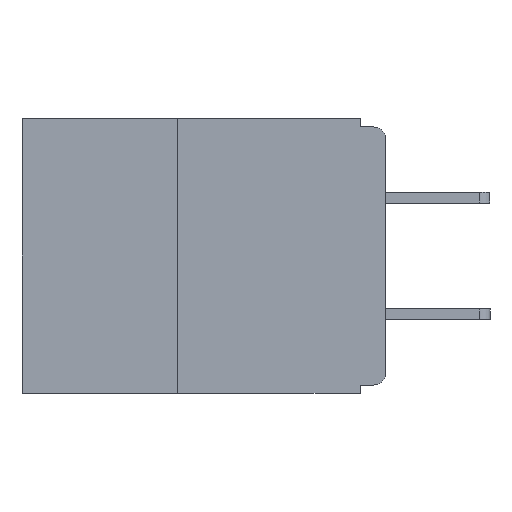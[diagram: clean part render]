
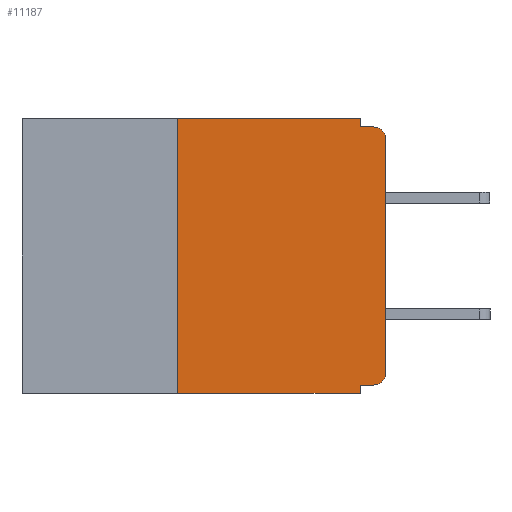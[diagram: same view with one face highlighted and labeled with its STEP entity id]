
A CAD part, left-side view. The second image highlights one B-rep face of the part: STEP entity #11187.
In plain terms, the highlighted planar face has unit normal (-1, 0, 0).
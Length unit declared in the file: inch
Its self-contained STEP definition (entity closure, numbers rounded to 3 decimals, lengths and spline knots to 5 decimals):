
#451 = EDGE_CURVE ( 'NONE', #9233, #1102, #5130, .T. ) ;
#1060 = CARTESIAN_POINT ( 'NONE',  ( 0., 0.437, 0. ) ) ;
#1102 = VERTEX_POINT ( 'NONE', #16081 ) ;
#1168 = VERTEX_POINT ( 'NONE', #16464 ) ;
#1625 = EDGE_LOOP ( 'NONE', ( #16126, #7980, #3937, #9539, #2246, #13802, #11364, #14177, #5556, #2811 ) ) ;
#1728 = EDGE_CURVE ( 'NONE', #16707, #11199, #4581, .T. ) ;
#2154 = LINE ( 'NONE', #1060, #18234 ) ;
#2246 = ORIENTED_EDGE ( 'NONE', *, *, #17163, .F. ) ;
#2491 = CARTESIAN_POINT ( 'NONE',  ( 0., 0.015, -0.32 ) ) ;
#2811 = ORIENTED_EDGE ( 'NONE', *, *, #14658, .T. ) ;
#3799 = CARTESIAN_POINT ( 'NONE',  ( 0., 0.015, -0.305 ) ) ;
#3903 = CARTESIAN_POINT ( 'NONE',  ( 0., 0., -0.01 ) ) ;
#3937 = ORIENTED_EDGE ( 'NONE', *, *, #18074, .F. ) ;
#4063 = DIRECTION ( 'NONE',  ( -1., 0., 0. ) ) ;
#4570 = DIRECTION ( 'NONE',  ( 0., 0., -1. ) ) ;
#4581 = LINE ( 'NONE', #18368, #12047 ) ;
#4763 = DIRECTION ( 'NONE',  ( 0., 0., -1. ) ) ;
#4775 = CARTESIAN_POINT ( 'NONE',  ( 0., 0.031, 0. ) ) ;
#4982 = CARTESIAN_POINT ( 'NONE',  ( 0., 0.015, -0.025 ) ) ;
#5008 = CARTESIAN_POINT ( 'NONE',  ( 0., 0., 0. ) ) ;
#5130 = LINE ( 'NONE', #5008, #12098 ) ;
#5236 = CARTESIAN_POINT ( 'NONE',  ( 0., 0., -0.305 ) ) ;
#5355 = DIRECTION ( 'NONE',  ( 0., 0., -1. ) ) ;
#5543 = LINE ( 'NONE', #8065, #14259 ) ;
#5556 = ORIENTED_EDGE ( 'NONE', *, *, #9085, .F. ) ;
#6046 = LINE ( 'NONE', #4775, #13821 ) ;
#6303 = CARTESIAN_POINT ( 'NONE',  ( 0., 0.25, -0.33 ) ) ;
#6414 = DIRECTION ( 'NONE',  ( 0., 0., 1. ) ) ;
#6687 = CARTESIAN_POINT ( 'NONE',  ( 0., 0.031, 0. ) ) ;
#6843 = CARTESIAN_POINT ( 'NONE',  ( 0., 0.031, -0.33 ) ) ;
#6888 = DIRECTION ( 'NONE',  ( 0., 0., -1. ) ) ;
#6938 = DIRECTION ( 'NONE',  ( 1., 0., 0. ) ) ;
#6985 = PLANE ( 'NONE',  #14329 ) ;
#7110 = CARTESIAN_POINT ( 'NONE',  ( 0., 0.437, 0. ) ) ;
#7200 = CARTESIAN_POINT ( 'NONE',  ( 0., 0.25, -0.33 ) ) ;
#7203 = LINE ( 'NONE', #6303, #14469 ) ;
#7341 = VERTEX_POINT ( 'NONE', #2491 ) ;
#7980 = ORIENTED_EDGE ( 'NONE', *, *, #8559, .T. ) ;
#8026 = DIRECTION ( 'NONE',  ( 0., 1., 0. ) ) ;
#8065 = CARTESIAN_POINT ( 'NONE',  ( 0., 0., -0.32 ) ) ;
#8151 = VERTEX_POINT ( 'NONE', #11420 ) ;
#8559 = EDGE_CURVE ( 'NONE', #1102, #12189, #18053, .T. ) ;
#9043 = DIRECTION ( 'NONE',  ( 0., 0., -1. ) ) ;
#9085 = EDGE_CURVE ( 'NONE', #7341, #17424, #5543, .T. ) ;
#9201 = EDGE_CURVE ( 'NONE', #16707, #8151, #7203, .T. ) ;
#9233 = VERTEX_POINT ( 'NONE', #5236 ) ;
#9539 = ORIENTED_EDGE ( 'NONE', *, *, #11335, .F. ) ;
#11187 = ADVANCED_FACE ( 'NONE', ( #16504 ), #6985, .F. ) ;
#11199 = VERTEX_POINT ( 'NONE', #6843 ) ;
#11335 = EDGE_CURVE ( 'NONE', #17496, #1168, #6046, .T. ) ;
#11364 = ORIENTED_EDGE ( 'NONE', *, *, #1728, .T. ) ;
#11420 = CARTESIAN_POINT ( 'NONE',  ( 0., 0.25, 0. ) ) ;
#11570 = DIRECTION ( 'NONE',  ( 0., -1., 0. ) ) ;
#12047 = VECTOR ( 'NONE', #18800, 39.37008 ) ;
#12098 = VECTOR ( 'NONE', #15264, 39.37008 ) ;
#12189 = VERTEX_POINT ( 'NONE', #13678 ) ;
#12194 = LINE ( 'NONE', #3903, #16413 ) ;
#12278 = CARTESIAN_POINT ( 'NONE',  ( 0., 0.031, -0.32 ) ) ;
#12390 = CIRCLE ( 'NONE', #17695, 0.015 ) ;
#12722 = AXIS2_PLACEMENT_3D ( 'NONE', #4982, #4063, #4763 ) ;
#12792 = DIRECTION ( 'NONE',  ( 0., -1., 0. ) ) ;
#13678 = CARTESIAN_POINT ( 'NONE',  ( 0., 0.015, -0.01 ) ) ;
#13802 = ORIENTED_EDGE ( 'NONE', *, *, #9201, .F. ) ;
#13821 = VECTOR ( 'NONE', #4570, 39.37008 ) ;
#14143 = DIRECTION ( 'NONE',  ( -1., 0., 0. ) ) ;
#14177 = ORIENTED_EDGE ( 'NONE', *, *, #17328, .F. ) ;
#14259 = VECTOR ( 'NONE', #8026, 39.37008 ) ;
#14329 = AXIS2_PLACEMENT_3D ( 'NONE', #7110, #6938, #6888 ) ;
#14469 = VECTOR ( 'NONE', #6414, 39.37008 ) ;
#14658 = EDGE_CURVE ( 'NONE', #7341, #9233, #12390, .T. ) ;
#15264 = DIRECTION ( 'NONE',  ( 0., 0., 1. ) ) ;
#15569 = VECTOR ( 'NONE', #9043, 39.37008 ) ;
#16081 = CARTESIAN_POINT ( 'NONE',  ( 0., 0., -0.025 ) ) ;
#16126 = ORIENTED_EDGE ( 'NONE', *, *, #451, .T. ) ;
#16413 = VECTOR ( 'NONE', #12792, 39.37008 ) ;
#16464 = CARTESIAN_POINT ( 'NONE',  ( 0., 0.031, -0.01 ) ) ;
#16504 = FACE_OUTER_BOUND ( 'NONE', #1625, .T. ) ;
#16707 = VERTEX_POINT ( 'NONE', #7200 ) ;
#17163 = EDGE_CURVE ( 'NONE', #8151, #17496, #2154, .T. ) ;
#17328 = EDGE_CURVE ( 'NONE', #17424, #11199, #18437, .T. ) ;
#17424 = VERTEX_POINT ( 'NONE', #12278 ) ;
#17496 = VERTEX_POINT ( 'NONE', #6687 ) ;
#17695 = AXIS2_PLACEMENT_3D ( 'NONE', #3799, #14143, #5355 ) ;
#17869 = CARTESIAN_POINT ( 'NONE',  ( 0., 0.031, -0.33 ) ) ;
#18053 = CIRCLE ( 'NONE', #12722, 0.015 ) ;
#18074 = EDGE_CURVE ( 'NONE', #1168, #12189, #12194, .T. ) ;
#18234 = VECTOR ( 'NONE', #11570, 39.37008 ) ;
#18368 = CARTESIAN_POINT ( 'NONE',  ( 0., 0.437, -0.33 ) ) ;
#18437 = LINE ( 'NONE', #17869, #15569 ) ;
#18800 = DIRECTION ( 'NONE',  ( 0., -1., 0. ) ) ;
